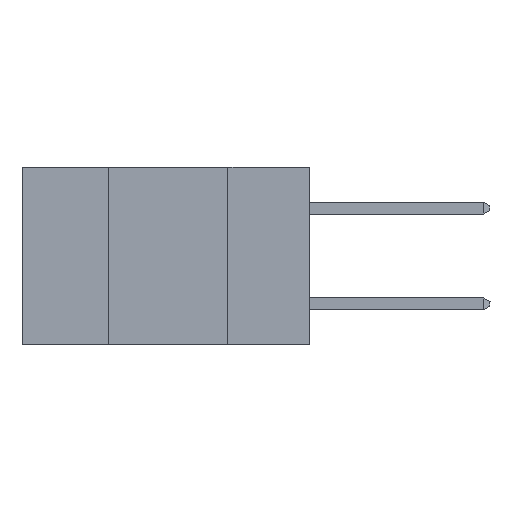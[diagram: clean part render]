
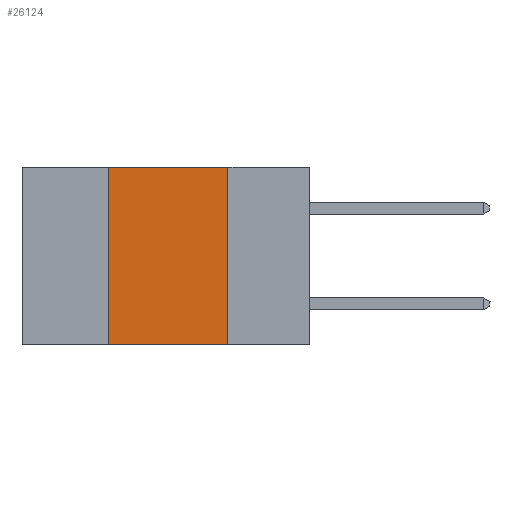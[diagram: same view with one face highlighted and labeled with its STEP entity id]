
A CAD part, left-side view. The second image highlights one B-rep face of the part: STEP entity #26124.
In plain terms, the highlighted planar face has unit normal (-1, 0, 0).
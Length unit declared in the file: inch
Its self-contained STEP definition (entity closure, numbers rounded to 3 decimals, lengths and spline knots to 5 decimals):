
#664 = AXIS2_PLACEMENT_3D ( 'NONE', #40566, #27785, #21117 ) ;
#1149 = ORIENTED_EDGE ( 'NONE', *, *, #11660, .F. ) ;
#2035 = ORIENTED_EDGE ( 'NONE', *, *, #15700, .F. ) ;
#3328 = VECTOR ( 'NONE', #26376, 39.37008 ) ;
#4388 = DIRECTION ( 'NONE',  ( 0., 0., -1. ) ) ;
#4487 = VERTEX_POINT ( 'NONE', #14214 ) ;
#5899 = CARTESIAN_POINT ( 'NONE',  ( 0., 0.17, 0. ) ) ;
#6651 = VECTOR ( 'NONE', #27352, 39.37008 ) ;
#7149 = VERTEX_POINT ( 'NONE', #41764 ) ;
#8697 = EDGE_CURVE ( 'NONE', #7149, #28761, #29933, .T. ) ;
#11299 = ORIENTED_EDGE ( 'NONE', *, *, #26068, .T. ) ;
#11660 = EDGE_CURVE ( 'NONE', #33578, #7149, #15359, .T. ) ;
#14214 = CARTESIAN_POINT ( 'NONE',  ( 0., 0.17, -0.37 ) ) ;
#14725 = VECTOR ( 'NONE', #40292, 39.37008 ) ;
#15359 = LINE ( 'NONE', #37029, #6651 ) ;
#15700 = EDGE_CURVE ( 'NONE', #28761, #4487, #32025, .T. ) ;
#16262 = ORIENTED_EDGE ( 'NONE', *, *, #8697, .F. ) ;
#16533 = CARTESIAN_POINT ( 'NONE',  ( 0., 0.6, 0. ) ) ;
#17281 = EDGE_LOOP ( 'NONE', ( #2035, #16262, #1149, #11299 ) ) ;
#18232 = PLANE ( 'NONE',  #664 ) ;
#21117 = DIRECTION ( 'NONE',  ( 0., 0., -1. ) ) ;
#23831 = CARTESIAN_POINT ( 'NONE',  ( 0., 0.6, -0.37 ) ) ;
#24937 = VECTOR ( 'NONE', #4388, 39.37008 ) ;
#26068 = EDGE_CURVE ( 'NONE', #33578, #4487, #31599, .T. ) ;
#26124 = ADVANCED_FACE ( 'NONE', ( #41748 ), #18232, .F. ) ;
#26376 = DIRECTION ( 'NONE',  ( 0., -1., 0. ) ) ;
#27352 = DIRECTION ( 'NONE',  ( 0., 0., 1. ) ) ;
#27785 = DIRECTION ( 'NONE',  ( 1., 0., 0. ) ) ;
#28761 = VERTEX_POINT ( 'NONE', #5899 ) ;
#29933 = LINE ( 'NONE', #16533, #3328 ) ;
#30256 = CARTESIAN_POINT ( 'NONE',  ( 0., 0.17, 0. ) ) ;
#31599 = LINE ( 'NONE', #23831, #14725 ) ;
#32025 = LINE ( 'NONE', #30256, #24937 ) ;
#33578 = VERTEX_POINT ( 'NONE', #38790 ) ;
#37029 = CARTESIAN_POINT ( 'NONE',  ( 0., 0.42, 0. ) ) ;
#38790 = CARTESIAN_POINT ( 'NONE',  ( 0., 0.42, -0.37 ) ) ;
#40292 = DIRECTION ( 'NONE',  ( 0., -1., 0. ) ) ;
#40566 = CARTESIAN_POINT ( 'NONE',  ( 0., 0.6, 0. ) ) ;
#41748 = FACE_OUTER_BOUND ( 'NONE', #17281, .T. ) ;
#41764 = CARTESIAN_POINT ( 'NONE',  ( 0., 0.42, 0. ) ) ;
